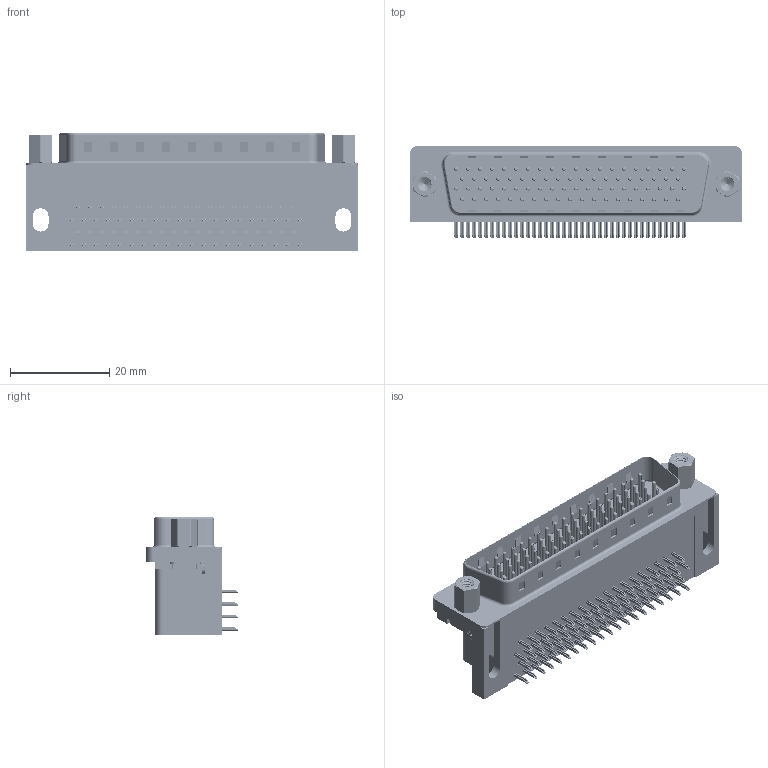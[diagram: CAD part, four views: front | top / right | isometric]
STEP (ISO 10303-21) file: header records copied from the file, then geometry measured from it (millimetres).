
FILE_DESCRIPTION (( 'STEP AP203' ), '1' );
FILE_NAME ('633-078-663-003.STEP', '2018-09-08T15:28:13', ( '' ), ( '' ), 'SwSTEP 2.0', 'SolidWorks 2016', '' );
FILE_SCHEMA (( 'CONFIG_CONTROL_DESIGN' ));
Length unit declared in the file: millimetre
Products named in the file (10): 633 Contact Top 78; 633 Non Board Mount_78 Contact; 633 4-40 Threaded Rivet; 633 4-40 Hex Standoff; 633 Housing_78 Contact; 633-078-663-003; 633 Shell_78 Contact; 633 Contact Bottom_78 Contact; 633 Contact Middle_78 Contact; 633 Contact Top_78 Contact
Assembly tree (86 placements, depth 2):
  633-078-663-003
    633 Housing_78 Contact
    633 Shell_78 Contact
    633 Contact Bottom_78 Contact  x19
    633 Contact Middle_78 Contact  x20
    633 Contact Top_78 Contact  x19
    633 Contact Top 78  x20
    633 Non Board Mount_78 Contact  x2
    633 4-40 Threaded Rivet  x2
    633 4-40 Hex Standoff  x2
Bounding box: 67 x 18.58 x 23.8 mm (x, y, z)
Volume: 14767.1 mm3; surface area: 16577.9 mm2
Topology: 86 solids, 86 shells, 6390 faces, 15724 edges, 9669 vertices
Faces by surface type: plane 4001, cylinder 1838, torus 499, cone 34, bspline 18
Entity records: 45471 total; most frequent: CARTESIAN_POINT 10904, DIRECTION 6608, ORIENTED_EDGE 6350, EDGE_CURVE 3175, VECTOR 2244, LINE 2244, AXIS2_PLACEMENT_3D 2182, VERTEX_POINT 2051
